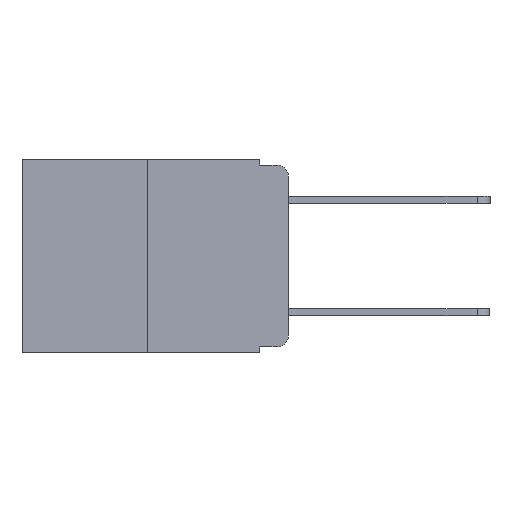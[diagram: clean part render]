
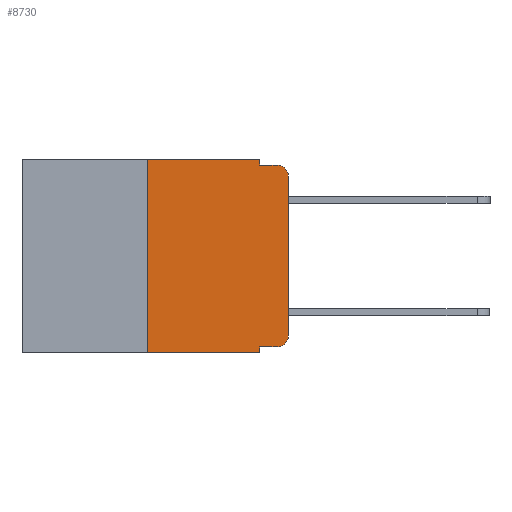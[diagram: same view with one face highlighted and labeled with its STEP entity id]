
A CAD part, left-side view. The second image highlights one B-rep face of the part: STEP entity #8730.
In plain terms, the highlighted planar face has unit normal (-1, 0, 0).
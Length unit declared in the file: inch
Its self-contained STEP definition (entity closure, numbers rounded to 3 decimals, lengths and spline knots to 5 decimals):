
#32 = VECTOR ( 'NONE', #2718, 39.37008 ) ;
#1050 = DIRECTION ( 'NONE',  ( 1., 0., 0. ) ) ;
#1395 = ORIENTED_EDGE ( 'NONE', *, *, #7347, .T. ) ;
#1805 = ORIENTED_EDGE ( 'NONE', *, *, #14189, .F. ) ;
#1898 = DIRECTION ( 'NONE',  ( 0., 0., 1. ) ) ;
#1901 = EDGE_CURVE ( 'NONE', #8942, #6776, #13258, .T. ) ;
#2083 = DIRECTION ( 'NONE',  ( 0., -1., 0. ) ) ;
#2396 = VECTOR ( 'NONE', #2083, 39.37008 ) ;
#2563 = ORIENTED_EDGE ( 'NONE', *, *, #9900, .F. ) ;
#2718 = DIRECTION ( 'NONE',  ( 0., 0., 1. ) ) ;
#2966 = LINE ( 'NONE', #12803, #8158 ) ;
#2989 = CARTESIAN_POINT ( 'NONE',  ( 0., 0.051, -0.333 ) ) ;
#3006 = CARTESIAN_POINT ( 'NONE',  ( 0., 0.051, -0.343 ) ) ;
#3049 = CARTESIAN_POINT ( 'NONE',  ( 0., 0.473, -0.343 ) ) ;
#3184 = CARTESIAN_POINT ( 'NONE',  ( 0., 0., 0. ) ) ;
#3409 = VECTOR ( 'NONE', #11124, 39.37008 ) ;
#3477 = AXIS2_PLACEMENT_3D ( 'NONE', #11661, #1050, #9513 ) ;
#3807 = LINE ( 'NONE', #3184, #6582 ) ;
#3850 = ORIENTED_EDGE ( 'NONE', *, *, #7674, .T. ) ;
#3875 = CARTESIAN_POINT ( 'NONE',  ( 0., 0.02, -0.313 ) ) ;
#3880 = ORIENTED_EDGE ( 'NONE', *, *, #1901, .F. ) ;
#4248 = VERTEX_POINT ( 'NONE', #4912 ) ;
#4296 = VECTOR ( 'NONE', #8077, 39.37008 ) ;
#4608 = ORIENTED_EDGE ( 'NONE', *, *, #14927, .T. ) ;
#4912 = CARTESIAN_POINT ( 'NONE',  ( 0., 0.25, -0.343 ) ) ;
#4932 = DIRECTION ( 'NONE',  ( 0., -1., 0. ) ) ;
#5073 = DIRECTION ( 'NONE',  ( 0., 0., -1. ) ) ;
#5137 = CARTESIAN_POINT ( 'NONE',  ( 0., 0.25, 0. ) ) ;
#6057 = DIRECTION ( 'NONE',  ( -1., 0., 0. ) ) ;
#6418 = VECTOR ( 'NONE', #11022, 39.37008 ) ;
#6423 = LINE ( 'NONE', #5137, #32 ) ;
#6582 = VECTOR ( 'NONE', #1898, 39.37008 ) ;
#6776 = VERTEX_POINT ( 'NONE', #10832 ) ;
#6913 = EDGE_CURVE ( 'NONE', #9322, #9508, #9823, .T. ) ;
#7205 = PLANE ( 'NONE',  #3477 ) ;
#7207 = VERTEX_POINT ( 'NONE', #11690 ) ;
#7347 = EDGE_CURVE ( 'NONE', #9508, #9159, #10515, .T. ) ;
#7441 = EDGE_LOOP ( 'NONE', ( #3850, #4608, #12071, #3880, #2563, #10621, #9445, #1805, #12984, #1395 ) ) ;
#7674 = EDGE_CURVE ( 'NONE', #9159, #15097, #3807, .T. ) ;
#8077 = DIRECTION ( 'NONE',  ( 0., 0., -1. ) ) ;
#8158 = VECTOR ( 'NONE', #4932, 39.37008 ) ;
#8686 = LINE ( 'NONE', #13515, #2396 ) ;
#8730 = ADVANCED_FACE ( 'NONE', ( #10275 ), #7205, .F. ) ;
#8942 = VERTEX_POINT ( 'NONE', #11977 ) ;
#8967 = CARTESIAN_POINT ( 'NONE',  ( 0., 0.051, 0. ) ) ;
#9057 = CARTESIAN_POINT ( 'NONE',  ( 0., 0., -0.313 ) ) ;
#9159 = VERTEX_POINT ( 'NONE', #9057 ) ;
#9322 = VERTEX_POINT ( 'NONE', #11450 ) ;
#9445 = ORIENTED_EDGE ( 'NONE', *, *, #14565, .T. ) ;
#9474 = VERTEX_POINT ( 'NONE', #3006 ) ;
#9508 = VERTEX_POINT ( 'NONE', #13256 ) ;
#9513 = DIRECTION ( 'NONE',  ( 0., 0., -1. ) ) ;
#9601 = VERTEX_POINT ( 'NONE', #14453 ) ;
#9624 = AXIS2_PLACEMENT_3D ( 'NONE', #3875, #11867, #5073 ) ;
#9823 = LINE ( 'NONE', #2989, #6418 ) ;
#9900 = EDGE_CURVE ( 'NONE', #9601, #8942, #2966, .T. ) ;
#10275 = FACE_OUTER_BOUND ( 'NONE', #7441, .T. ) ;
#10396 = EDGE_CURVE ( 'NONE', #6776, #7207, #8686, .T. ) ;
#10515 = CIRCLE ( 'NONE', #9624, 0.02 ) ;
#10621 = ORIENTED_EDGE ( 'NONE', *, *, #15068, .F. ) ;
#10832 = CARTESIAN_POINT ( 'NONE',  ( 0., 0.051, -0.01 ) ) ;
#10867 = CIRCLE ( 'NONE', #15108, 0.02 ) ;
#10872 = CARTESIAN_POINT ( 'NONE',  ( 0., 0., -0.03 ) ) ;
#11022 = DIRECTION ( 'NONE',  ( 0., -1., 0. ) ) ;
#11124 = DIRECTION ( 'NONE',  ( 0., -1., 0. ) ) ;
#11168 = LINE ( 'NONE', #12636, #13654 ) ;
#11450 = CARTESIAN_POINT ( 'NONE',  ( 0., 0.051, -0.333 ) ) ;
#11661 = CARTESIAN_POINT ( 'NONE',  ( 0., 0.473, 0. ) ) ;
#11690 = CARTESIAN_POINT ( 'NONE',  ( 0., 0.02, -0.01 ) ) ;
#11867 = DIRECTION ( 'NONE',  ( -1., 0., 0. ) ) ;
#11977 = CARTESIAN_POINT ( 'NONE',  ( 0., 0.051, 0. ) ) ;
#12071 = ORIENTED_EDGE ( 'NONE', *, *, #10396, .F. ) ;
#12169 = LINE ( 'NONE', #3049, #3409 ) ;
#12636 = CARTESIAN_POINT ( 'NONE',  ( 0., 0.051, 0. ) ) ;
#12753 = CARTESIAN_POINT ( 'NONE',  ( 0., 0.02, -0.03 ) ) ;
#12803 = CARTESIAN_POINT ( 'NONE',  ( 0., 0.473, 0. ) ) ;
#12984 = ORIENTED_EDGE ( 'NONE', *, *, #6913, .T. ) ;
#13256 = CARTESIAN_POINT ( 'NONE',  ( 0., 0.02, -0.333 ) ) ;
#13258 = LINE ( 'NONE', #8967, #4296 ) ;
#13515 = CARTESIAN_POINT ( 'NONE',  ( 0., 0.051, -0.01 ) ) ;
#13654 = VECTOR ( 'NONE', #14730, 39.37008 ) ;
#13810 = DIRECTION ( 'NONE',  ( 0., 0., -1. ) ) ;
#14189 = EDGE_CURVE ( 'NONE', #9322, #9474, #11168, .T. ) ;
#14453 = CARTESIAN_POINT ( 'NONE',  ( 0., 0.25, 0. ) ) ;
#14565 = EDGE_CURVE ( 'NONE', #4248, #9474, #12169, .T. ) ;
#14730 = DIRECTION ( 'NONE',  ( 0., 0., -1. ) ) ;
#14927 = EDGE_CURVE ( 'NONE', #15097, #7207, #10867, .T. ) ;
#15068 = EDGE_CURVE ( 'NONE', #4248, #9601, #6423, .T. ) ;
#15097 = VERTEX_POINT ( 'NONE', #10872 ) ;
#15108 = AXIS2_PLACEMENT_3D ( 'NONE', #12753, #6057, #13810 ) ;
